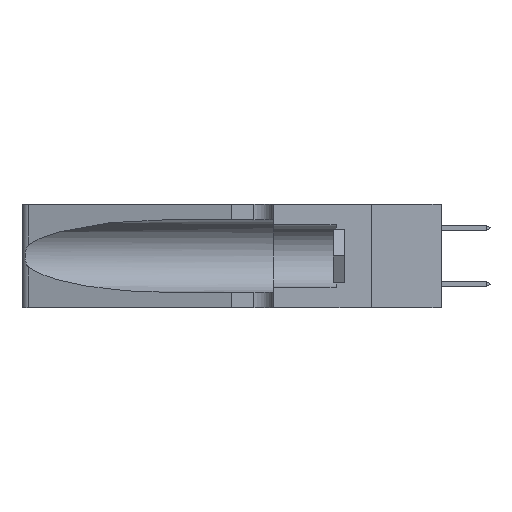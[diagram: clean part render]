
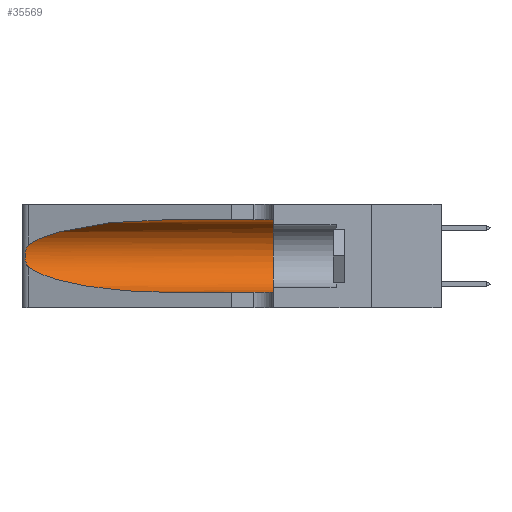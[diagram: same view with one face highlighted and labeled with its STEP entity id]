
A CAD part, left-side view. The second image highlights one B-rep face of the part: STEP entity #35569.
In plain terms, the highlighted cylindrical face has radius 3.308 mm (diameter 6.617 mm), a partial arc.
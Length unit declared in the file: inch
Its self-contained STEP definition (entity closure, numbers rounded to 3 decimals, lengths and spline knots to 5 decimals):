
#346 = DIRECTION ( 'NONE',  ( 0., 0., -1. ) ) ;
#701 = CYLINDRICAL_SURFACE ( 'NONE', #42930, 0.13025 ) ;
#1851 = LINE ( 'NONE', #9912, #20063 ) ;
#1878 = CARTESIAN_POINT ( 'NONE',  ( 0.1305, 0.72297, 0.31525 ) ) ;
#2071 = ORIENTED_EDGE ( 'NONE', *, *, #41096, .T. ) ;
#2494 = CARTESIAN_POINT ( 'NONE',  ( 0.25854, 1.2359, 0.20912 ) ) ;
#2754 =( BOUNDED_CURVE ( )  B_SPLINE_CURVE ( 3, ( #40752, #34151, #27529, #7157 ),
 .UNSPECIFIED., .F., .T. ) 
 B_SPLINE_CURVE_WITH_KNOTS ( ( 4, 4 ),
 ( 3.44316, 4.71239 ),
 .UNSPECIFIED. ) 
 CURVE ( )  GEOMETRIC_REPRESENTATION_ITEM ( )  RATIONAL_B_SPLINE_CURVE ( ( 1., 0.87, 0.87, 1. ) ) 
 REPRESENTATION_ITEM ( '' )  );
#3291 = ORIENTED_EDGE ( 'NONE', *, *, #3900, .T. ) ;
#3663 = ORIENTED_EDGE ( 'NONE', *, *, #28417, .T. ) ;
#3900 = EDGE_CURVE ( 'NONE', #11579, #41877, #14045, .T. ) ;
#4368 = ORIENTED_EDGE ( 'NONE', *, *, #9395, .T. ) ;
#5762 = ORIENTED_EDGE ( 'NONE', *, *, #34386, .F. ) ;
#5950 = CARTESIAN_POINT ( 'NONE',  ( 0.26075, 1.23896, 0.19203 ) ) ;
#6640 = CARTESIAN_POINT ( 'NONE',  ( 0.1305, 0.72297, 0.31525 ) ) ;
#7157 = CARTESIAN_POINT ( 'NONE',  ( 0.1305, 0.72297, 0.05475 ) ) ;
#7829 = CIRCLE ( 'NONE', #32158, 0.13025 ) ;
#7935 = ORIENTED_EDGE ( 'NONE', *, *, #41741, .F. ) ;
#9238 = EDGE_LOOP ( 'NONE', ( #2071, #3291, #3663, #4368, #5762, #7935 ) ) ;
#9395 = EDGE_CURVE ( 'NONE', #23797, #16886, #24257, .T. ) ;
#9437 = CARTESIAN_POINT ( 'NONE',  ( 0.26017, 1.23833, 0.17102 ) ) ;
#9912 = CARTESIAN_POINT ( 'NONE',  ( 0.1305, 1.61858, 0.31525 ) ) ;
#10102 = CARTESIAN_POINT ( 'NONE',  ( 0.18966, 0.96281, 0.31525 ) ) ;
#11579 = VERTEX_POINT ( 'NONE', #24513 ) ;
#12850 = CARTESIAN_POINT ( 'NONE',  ( 0.25789, 1.23486, 0.15765 ) ) ;
#13541 = CARTESIAN_POINT ( 'NONE',  ( 0.25487, 1.22718, 0.22369 ) ) ;
#14045 = B_SPLINE_CURVE_WITH_KNOTS ( 'NONE', 3,
 ( #42890, #19567, #16164, #22952, #2494, #26343, #5950, #29738, #9437, #33143, #12850, #36439, #16302, #39751 ),
 .UNSPECIFIED., .F., .F.,
 ( 4, 2, 2, 2, 2, 2, 4 ),
 ( 0., 0.00027, 0.00053, 0.00107, 0.0016, 0.00187, 0.00214 ),
 .UNSPECIFIED. ) ;
#14566 = DIRECTION ( 'NONE',  ( 0., 1., 0. ) ) ;
#16164 = CARTESIAN_POINT ( 'NONE',  ( 0.25639, 1.23184, 0.21858 ) ) ;
#16302 = CARTESIAN_POINT ( 'NONE',  ( 0.25555, 1.22993, 0.14849 ) ) ;
#16854 = CARTESIAN_POINT ( 'NONE',  ( 0.1305, 1.61858, 0.05475 ) ) ;
#16886 = VERTEX_POINT ( 'NONE', #41567 ) ;
#17594 = DIRECTION ( 'NONE',  ( 0., -1., 0. ) ) ;
#19567 = CARTESIAN_POINT ( 'NONE',  ( 0.25555, 1.22994, 0.2215 ) ) ;
#20063 = VECTOR ( 'NONE', #33596, 39.37008 ) ;
#20266 = DIRECTION ( 'NONE',  ( 0., -1., 0. ) ) ;
#22139 = CARTESIAN_POINT ( 'NONE',  ( 0.1305, 0.72297, 0.05475 ) ) ;
#22952 = CARTESIAN_POINT ( 'NONE',  ( 0.25787, 1.23484, 0.2124 ) ) ;
#23210 = VECTOR ( 'NONE', #20266, 39.37008 ) ;
#23227 = CARTESIAN_POINT ( 'NONE',  ( 0.1305, 0.35, 0.31525 ) ) ;
#23797 = VERTEX_POINT ( 'NONE', #22139 ) ;
#24257 = LINE ( 'NONE', #16854, #23210 ) ;
#24513 = CARTESIAN_POINT ( 'NONE',  ( 0.25487, 1.22718, 0.22369 ) ) ;
#25129 = VERTEX_POINT ( 'NONE', #1878 ) ;
#26343 = CARTESIAN_POINT ( 'NONE',  ( 0.26018, 1.23835, 0.19895 ) ) ;
#27127 = VERTEX_POINT ( 'NONE', #23227 ) ;
#27529 = CARTESIAN_POINT ( 'NONE',  ( 0.18966, 0.96281, 0.05475 ) ) ;
#27683 = CARTESIAN_POINT ( 'NONE',  ( 0.25487, 1.22718, 0.14631 ) ) ;
#28417 = EDGE_CURVE ( 'NONE', #41877, #23797, #2754, .T. ) ;
#29738 = CARTESIAN_POINT ( 'NONE',  ( 0.26075, 1.23896, 0.178 ) ) ;
#32158 = AXIS2_PLACEMENT_3D ( 'NONE', #34740, #14566, #38046 ) ;
#33143 = CARTESIAN_POINT ( 'NONE',  ( 0.25856, 1.23593, 0.16098 ) ) ;
#33596 = DIRECTION ( 'NONE',  ( 0., -1., 0. ) ) ;
#33789 = CARTESIAN_POINT ( 'NONE',  ( 0.2373, 1.15595, 0.28018 ) ) ;
#34151 = CARTESIAN_POINT ( 'NONE',  ( 0.2373, 1.15595, 0.08982 ) ) ;
#34386 = EDGE_CURVE ( 'NONE', #27127, #16886, #7829, .T. ) ;
#34740 = CARTESIAN_POINT ( 'NONE',  ( 0.1305, 0.35, 0.185 ) ) ;
#35569 = ADVANCED_FACE ( 'NONE', ( #36795 ), #701, .F. ) ;
#35641 =( BOUNDED_CURVE ( )  B_SPLINE_CURVE ( 3, ( #6640, #10102, #33789, #13541 ),
 .UNSPECIFIED., .F., .F. ) 
 B_SPLINE_CURVE_WITH_KNOTS ( ( 4, 4 ),
 ( 1.5708, 2.84003 ),
 .UNSPECIFIED. ) 
 CURVE ( )  GEOMETRIC_REPRESENTATION_ITEM ( )  RATIONAL_B_SPLINE_CURVE ( ( 1., 0.87, 0.87, 1. ) ) 
 REPRESENTATION_ITEM ( '' )  );
#36439 = CARTESIAN_POINT ( 'NONE',  ( 0.25639, 1.23186, 0.15144 ) ) ;
#36795 = FACE_OUTER_BOUND ( 'NONE', #9238, .T. ) ;
#38046 = DIRECTION ( 'NONE',  ( 0., 0., 1. ) ) ;
#39751 = CARTESIAN_POINT ( 'NONE',  ( 0.25487, 1.22718, 0.14631 ) ) ;
#40752 = CARTESIAN_POINT ( 'NONE',  ( 0.25487, 1.22718, 0.14631 ) ) ;
#40990 = CARTESIAN_POINT ( 'NONE',  ( 0.1305, 1.61858, 0.185 ) ) ;
#41096 = EDGE_CURVE ( 'NONE', #25129, #11579, #35641, .T. ) ;
#41567 = CARTESIAN_POINT ( 'NONE',  ( 0.1305, 0.35, 0.05475 ) ) ;
#41741 = EDGE_CURVE ( 'NONE', #25129, #27127, #1851, .T. ) ;
#41877 = VERTEX_POINT ( 'NONE', #27683 ) ;
#42890 = CARTESIAN_POINT ( 'NONE',  ( 0.25487, 1.22718, 0.22369 ) ) ;
#42930 = AXIS2_PLACEMENT_3D ( 'NONE', #40990, #17594, #346 ) ;
